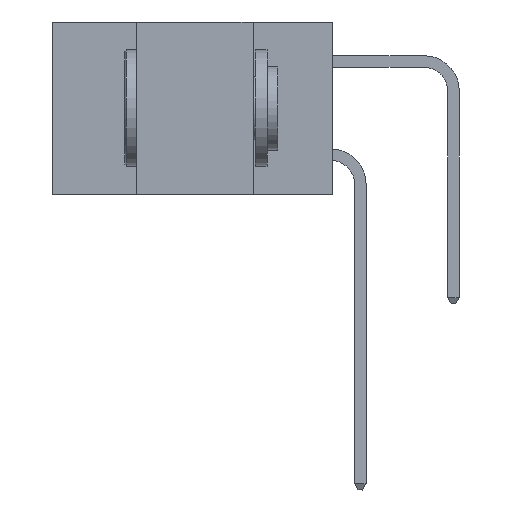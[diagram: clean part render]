
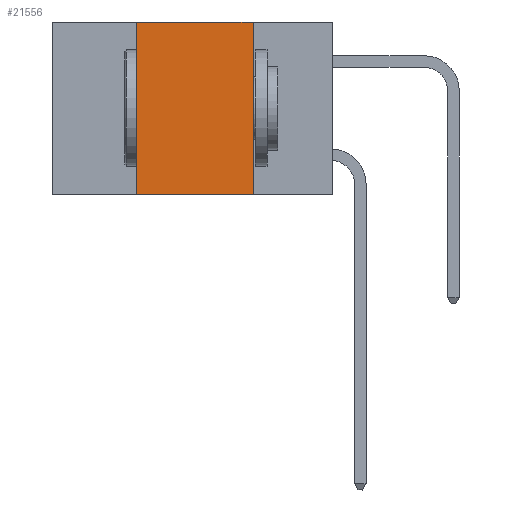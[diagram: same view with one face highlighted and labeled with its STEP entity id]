
A CAD part, left-side view. The second image highlights one B-rep face of the part: STEP entity #21556.
In plain terms, the highlighted planar face has unit normal (-1, 0, 0).
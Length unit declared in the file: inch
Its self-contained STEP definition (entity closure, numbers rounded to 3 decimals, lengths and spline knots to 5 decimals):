
#336 = ORIENTED_EDGE ( 'NONE', *, *, #3807, .F. ) ;
#719 = CARTESIAN_POINT ( 'NONE',  ( 0., 0.17, -0.37 ) ) ;
#1119 = ORIENTED_EDGE ( 'NONE', *, *, #5425, .T. ) ;
#3193 = AXIS2_PLACEMENT_3D ( 'NONE', #9643, #9407, #6295 ) ;
#3381 = EDGE_LOOP ( 'NONE', ( #336, #13766, #12506, #1119 ) ) ;
#3807 = EDGE_CURVE ( 'NONE', #14471, #21469, #4562, .T. ) ;
#4562 = LINE ( 'NONE', #15146, #10267 ) ;
#4638 = VECTOR ( 'NONE', #10031, 39.37008 ) ;
#5425 = EDGE_CURVE ( 'NONE', #18014, #21469, #8812, .T. ) ;
#5449 = CARTESIAN_POINT ( 'NONE',  ( 0., 0.42, -0.37 ) ) ;
#5483 = CARTESIAN_POINT ( 'NONE',  ( 0., 0.6, -0.37 ) ) ;
#6295 = DIRECTION ( 'NONE',  ( 0., 0., -1. ) ) ;
#8482 = VECTOR ( 'NONE', #21840, 39.37008 ) ;
#8614 = CARTESIAN_POINT ( 'NONE',  ( 0., 0.17, 0. ) ) ;
#8641 = VERTEX_POINT ( 'NONE', #14882 ) ;
#8812 = LINE ( 'NONE', #5483, #9161 ) ;
#9161 = VECTOR ( 'NONE', #14517, 39.37008 ) ;
#9407 = DIRECTION ( 'NONE',  ( 1., 0., 0. ) ) ;
#9643 = CARTESIAN_POINT ( 'NONE',  ( 0., 0.6, 0. ) ) ;
#10031 = DIRECTION ( 'NONE',  ( 0., -1., 0. ) ) ;
#10267 = VECTOR ( 'NONE', #22501, 39.37008 ) ;
#12227 = LINE ( 'NONE', #5449, #8482 ) ;
#12316 = CARTESIAN_POINT ( 'NONE',  ( 0., 0.42, -0.37 ) ) ;
#12506 = ORIENTED_EDGE ( 'NONE', *, *, #17610, .F. ) ;
#13766 = ORIENTED_EDGE ( 'NONE', *, *, #19355, .F. ) ;
#14053 = LINE ( 'NONE', #23075, #4638 ) ;
#14471 = VERTEX_POINT ( 'NONE', #8614 ) ;
#14517 = DIRECTION ( 'NONE',  ( 0., -1., 0. ) ) ;
#14882 = CARTESIAN_POINT ( 'NONE',  ( 0., 0.42, 0. ) ) ;
#15146 = CARTESIAN_POINT ( 'NONE',  ( 0., 0.17, -0.37 ) ) ;
#15218 = PLANE ( 'NONE',  #3193 ) ;
#17610 = EDGE_CURVE ( 'NONE', #18014, #8641, #12227, .T. ) ;
#18014 = VERTEX_POINT ( 'NONE', #12316 ) ;
#18441 = FACE_OUTER_BOUND ( 'NONE', #3381, .T. ) ;
#19355 = EDGE_CURVE ( 'NONE', #8641, #14471, #14053, .T. ) ;
#21469 = VERTEX_POINT ( 'NONE', #719 ) ;
#21556 = ADVANCED_FACE ( 'NONE', ( #18441 ), #15218, .F. ) ;
#21840 = DIRECTION ( 'NONE',  ( 0., 0., 1. ) ) ;
#22501 = DIRECTION ( 'NONE',  ( 0., 0., -1. ) ) ;
#23075 = CARTESIAN_POINT ( 'NONE',  ( 0., 0.6, 0. ) ) ;
